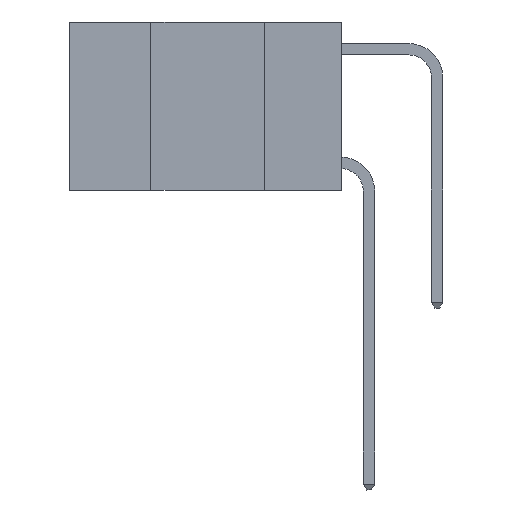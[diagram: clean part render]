
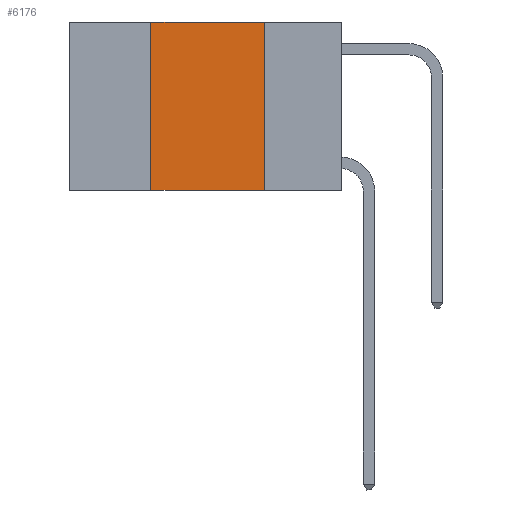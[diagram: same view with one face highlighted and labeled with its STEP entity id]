
A CAD part, left-side view. The second image highlights one B-rep face of the part: STEP entity #6176.
In plain terms, the highlighted planar face has unit normal (-1, 0, 0).
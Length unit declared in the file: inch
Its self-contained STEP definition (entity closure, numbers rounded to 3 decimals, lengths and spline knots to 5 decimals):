
#1184 = EDGE_LOOP ( 'NONE', ( #2493, #10296, #5516, #11270 ) ) ;
#1417 = DIRECTION ( 'NONE',  ( 0., 0., -1. ) ) ;
#1460 = CARTESIAN_POINT ( 'NONE',  ( 0., 0.6, 0. ) ) ;
#1625 = DIRECTION ( 'NONE',  ( 1., 0., 0. ) ) ;
#1855 = CARTESIAN_POINT ( 'NONE',  ( 0., 0.42, 0. ) ) ;
#2224 = CARTESIAN_POINT ( 'NONE',  ( 0., 0.17, -0.37 ) ) ;
#2493 = ORIENTED_EDGE ( 'NONE', *, *, #5684, .F. ) ;
#2725 = VECTOR ( 'NONE', #6840, 39.37008 ) ;
#3094 = LINE ( 'NONE', #9322, #9478 ) ;
#3140 = VERTEX_POINT ( 'NONE', #1855 ) ;
#3584 = PLANE ( 'NONE',  #9086 ) ;
#4574 = DIRECTION ( 'NONE',  ( 0., -1., 0. ) ) ;
#5448 = EDGE_CURVE ( 'NONE', #3140, #9835, #10998, .T. ) ;
#5516 = ORIENTED_EDGE ( 'NONE', *, *, #6273, .F. ) ;
#5684 = EDGE_CURVE ( 'NONE', #9835, #6832, #8719, .T. ) ;
#6109 = LINE ( 'NONE', #7002, #9569 ) ;
#6176 = ADVANCED_FACE ( 'NONE', ( #8761 ), #3584, .F. ) ;
#6273 = EDGE_CURVE ( 'NONE', #10018, #3140, #6109, .T. ) ;
#6336 = DIRECTION ( 'NONE',  ( 0., -1., 0. ) ) ;
#6420 = CARTESIAN_POINT ( 'NONE',  ( 0., 0.17, 0. ) ) ;
#6628 = CARTESIAN_POINT ( 'NONE',  ( 0., 0.17, 0. ) ) ;
#6832 = VERTEX_POINT ( 'NONE', #2224 ) ;
#6840 = DIRECTION ( 'NONE',  ( 0., 0., -1. ) ) ;
#7002 = CARTESIAN_POINT ( 'NONE',  ( 0., 0.42, 0. ) ) ;
#7593 = VECTOR ( 'NONE', #4574, 39.37008 ) ;
#8509 = EDGE_CURVE ( 'NONE', #10018, #6832, #3094, .T. ) ;
#8719 = LINE ( 'NONE', #6628, #2725 ) ;
#8761 = FACE_OUTER_BOUND ( 'NONE', #1184, .T. ) ;
#9086 = AXIS2_PLACEMENT_3D ( 'NONE', #11916, #1625, #1417 ) ;
#9322 = CARTESIAN_POINT ( 'NONE',  ( 0., 0.6, -0.37 ) ) ;
#9478 = VECTOR ( 'NONE', #6336, 39.37008 ) ;
#9569 = VECTOR ( 'NONE', #10456, 39.37008 ) ;
#9835 = VERTEX_POINT ( 'NONE', #6420 ) ;
#10018 = VERTEX_POINT ( 'NONE', #13201 ) ;
#10296 = ORIENTED_EDGE ( 'NONE', *, *, #5448, .F. ) ;
#10456 = DIRECTION ( 'NONE',  ( 0., 0., 1. ) ) ;
#10998 = LINE ( 'NONE', #1460, #7593 ) ;
#11270 = ORIENTED_EDGE ( 'NONE', *, *, #8509, .T. ) ;
#11916 = CARTESIAN_POINT ( 'NONE',  ( 0., 0.6, 0. ) ) ;
#13201 = CARTESIAN_POINT ( 'NONE',  ( 0., 0.42, -0.37 ) ) ;
